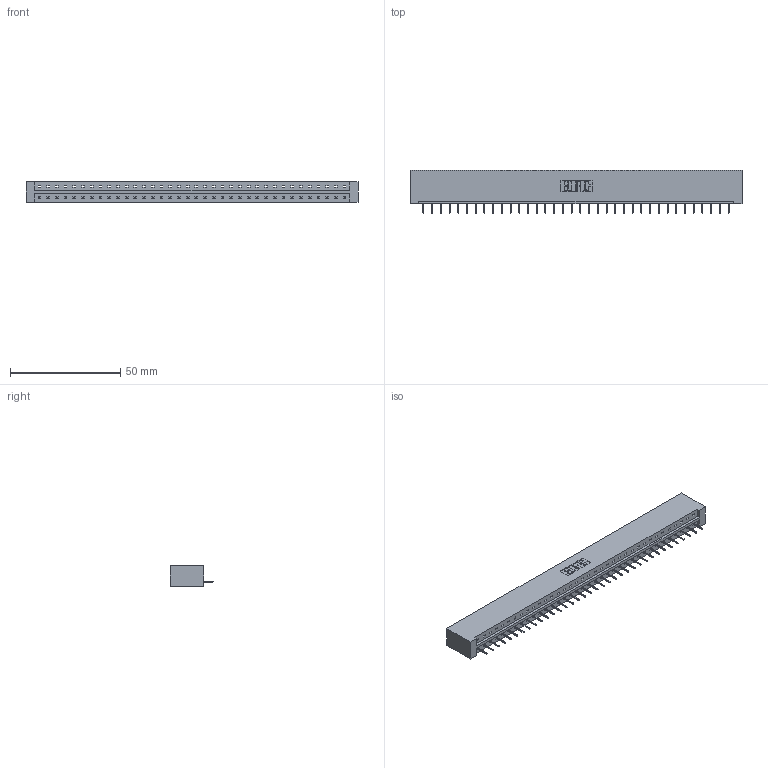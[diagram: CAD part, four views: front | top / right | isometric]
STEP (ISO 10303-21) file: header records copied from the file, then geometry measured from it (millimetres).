
FILE_DESCRIPTION (( 'STEP AP203' ), '1' );
FILE_NAME ('333-036-524-101.STEP', '2018-08-03T00:40:51', ( '' ), ( '' ), 'SwSTEP 2.0', 'SolidWorks 2016', '' );
FILE_SCHEMA (( 'CONFIG_CONTROL_DESIGN' ));
Length unit declared in the file: inch
Products named in the file (3): 333 Part_Lugless; 345-292-001_345-293-124; 333-036-524-101
Assembly tree (37 placements, depth 2):
  333-036-524-101
    333 Part_Lugless
    345-292-001_345-293-124  x36
Bounding box: 150.9 x 19.69 x 9.4 mm (x, y, z)
Volume: 15603.9 mm3; surface area: 16311.7 mm2
Topology: 37 solids, 37 shells, 2338 faces, 6767 edges, 4366 vertices
Faces by surface type: plane 1794, cylinder 544
Entity records: 22581 total; most frequent: CARTESIAN_POINT 3902, ORIENTED_EDGE 3874, DIRECTION 3297, EDGE_CURVE 1937, VECTOR 1821, LINE 1821, VERTEX_POINT 1286, AXIS2_PLACEMENT_3D 738
